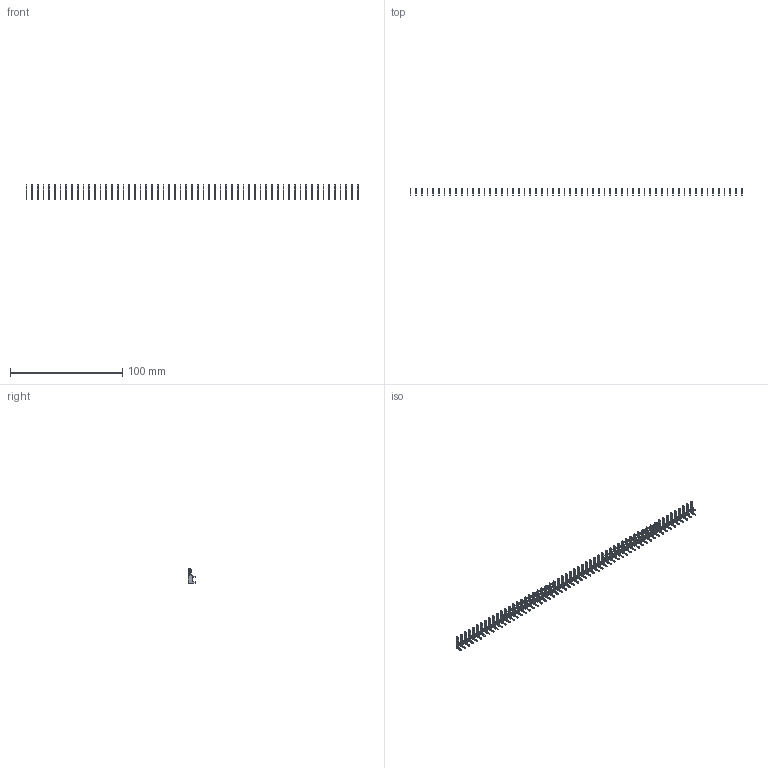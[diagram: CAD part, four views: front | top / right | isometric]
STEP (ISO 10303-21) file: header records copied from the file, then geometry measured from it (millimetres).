
FILE_DESCRIPTION (( 'STEP AP203' ), '1' );
FILE_NAME ('105-059-203-200.STEP', '2020-08-30T00:35:22', ( '' ), ( '' ), 'SwSTEP 2.0', 'SolidWorks 2020', '' );
FILE_SCHEMA (( 'CONFIG_CONTROL_DESIGN' ));
Length unit declared in the file: inch
Products named in the file (2): 105-059-203-200; 100-290-001_100-290-203
Assembly tree (59 placements, depth 2):
  105-059-203-200
    100-290-001_100-290-203  x59
Bounding box: 295.24 x 6.52 x 12.7 mm (x, y, z)
Volume: 1489.5 mm3; surface area: 6827.4 mm2
Topology: 59 solids, 59 shells, 1652 faces, 4602 edges, 3068 vertices
Faces by surface type: plane 1239, cylinder 413
Entity records: 2952 total; most frequent: DIRECTION 268, CARTESIAN_POINT 232, ORIENTED_EDGE 156, LOCAL_TIME 128, DATE_AND_TIME 128, COORDINATED_UNIVERSAL_TIME_OFFSET 128, CALENDAR_DATE 128, AXIS2_PLACEMENT_3D 104
